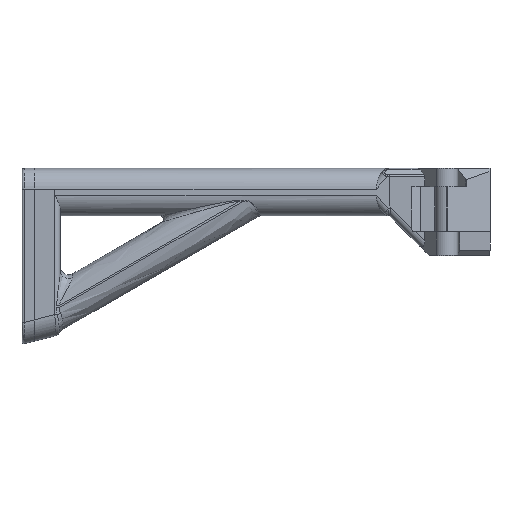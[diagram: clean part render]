
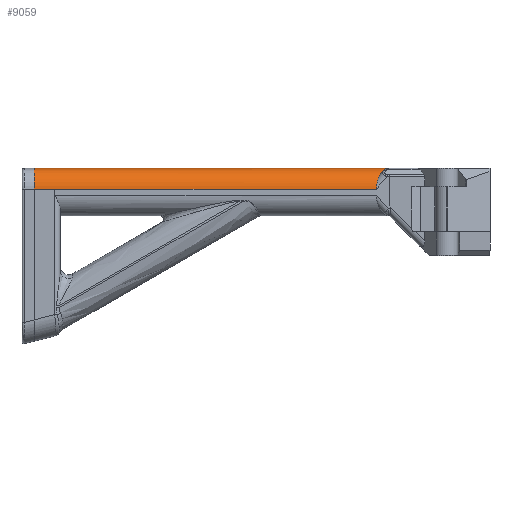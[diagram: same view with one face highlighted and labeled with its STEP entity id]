
A CAD part, top view. The second image highlights one B-rep face of the part: STEP entity #9059.
In plain terms, the highlighted cylindrical face has radius 12 mm (diameter 24 mm), a partial arc.
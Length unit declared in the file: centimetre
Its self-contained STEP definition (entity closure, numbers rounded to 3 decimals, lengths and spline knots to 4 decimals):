
#76=ELLIPSE($,#9789,1.6091,1.2);
#812=LINE($,#16482,#1668);
#829=LINE($,#16588,#1685);
#942=LINE($,#18000,#1798);
#1668=VECTOR($,#12061,18.606);
#1685=VECTOR($,#12090,20.5279);
#1798=VECTOR($,#12463,1.2);
#2109=B_SPLINE_CURVE_WITH_KNOTS($,3,(#16510,#16511,#16512,#16513,#16514,
#16515,#16516,#16517,#16518,#16519,#16520,#16521,#16522,#16523,#16524,#16525,
#16526,#16527,#16528,#16529,#16530,#16531,#16532,#16533,#16534,#16535,#16536,
#16537,#16538,#16539,#16540,#16541,#16542,#16543,#16544,#16545,#16546,#16547,
#16548,#16549,#16550,#16551,#16552,#16553,#16554,#16555,#16556,#16557),
 .UNSPECIFIED.,.F.,.F.,(4,2,2,2,2,2,2,2,2,2,2,2,2,2,2,2,2,2,2,2,2,2,2,4),
(2.2553,2.2555,2.2557,2.256,2.2565,
2.257,2.2583,2.2596,2.2621,2.2699,
2.2857,2.3174,2.3491,2.3808,2.444,
2.5071,2.5694,2.6316,2.6939,2.7562,
2.8753,2.9944,3.1135,3.2326),
 .UNSPECIFIED.);
#2110=B_SPLINE_CURVE_WITH_KNOTS($,3,(#16565,#16566,#16567,#16568,#16569,
#16570),.UNSPECIFIED.,.F.,.F.,(4,2,4),(2.7496,2.9106,
3.3544),.UNSPECIFIED.);
#2744=FACE_OUTER_BOUND($,#3293,.T.);
#3293=EDGE_LOOP($,(#8300,#8301,#8302,#8303,#8304,#8305,#8306,#8307));
#3648=CIRCLE($,#9931,1.2);
#3649=CIRCLE($,#9932,1.2);
#4307=VERTEX_POINT($,#16479);
#4308=VERTEX_POINT($,#16481);
#4315=VERTEX_POINT($,#16508);
#4316=VERTEX_POINT($,#16559);
#4317=VERTEX_POINT($,#16563);
#4325=VERTEX_POINT($,#16586);
#4456=VERTEX_POINT($,#17996);
#4458=VERTEX_POINT($,#17999);
#5508=EDGE_CURVE($,#4308,#4307,#812,.F.);
#5517=EDGE_CURVE($,#4315,#4307,#2109,.F.);
#5519=EDGE_CURVE($,#4315,#4316,#76,.F.);
#5521=EDGE_CURVE($,#4317,#4316,#2110,.F.);
#5530=EDGE_CURVE($,#4317,#4325,#829,.T.);
#5740=EDGE_CURVE($,#4458,#4456,#942,.T.);
#5757=EDGE_CURVE($,#4325,#4458,#3648,.F.);
#5758=EDGE_CURVE($,#4308,#4456,#3649,.T.);
#8300=ORIENTED_EDGE($,*,*,#5508,.T.);
#8301=ORIENTED_EDGE($,*,*,#5517,.F.);
#8302=ORIENTED_EDGE($,*,*,#5519,.T.);
#8303=ORIENTED_EDGE($,*,*,#5521,.F.);
#8304=ORIENTED_EDGE($,*,*,#5530,.T.);
#8305=ORIENTED_EDGE($,*,*,#5757,.T.);
#8306=ORIENTED_EDGE($,*,*,#5740,.T.);
#8307=ORIENTED_EDGE($,*,*,#5758,.F.);
#8557=CYLINDRICAL_SURFACE($,#9930,1.2);
#9059=ADVANCED_FACE($,(#2744),#8557,.T.);
#9789=AXIS2_PLACEMENT_3D($,#16561,#12074,#12075);
#9930=AXIS2_PLACEMENT_3D($,#18053,#12486,#12487);
#9931=AXIS2_PLACEMENT_3D($,#18054,#12488,#12489);
#9932=AXIS2_PLACEMENT_3D($,#18055,#12490,#12491);
#12061=DIRECTION($,(-1.,0.,0.));
#12074=DIRECTION('center_axis',(0.746,-0.666,0.));
#12075=DIRECTION('ref_axis',(0.666,0.746,0.));
#12090=DIRECTION($,(-1.,0.,0.));
#12463=DIRECTION($,(1.,0.,0.));
#12486=DIRECTION('center_axis',(1.,0.,0.));
#12487=DIRECTION('ref_axis',(0.,0.707,0.707));
#12488=DIRECTION('center_axis',(-1.,0.,0.));
#12489=DIRECTION('ref_axis',(0.,0.707,0.707));
#12490=DIRECTION('center_axis',(1.,0.,0.));
#12491=DIRECTION('ref_axis',(0.,0.707,0.707));
#16479=CARTESIAN_POINT('',(-26.3838,3.902,4.4797));
#16481=CARTESIAN_POINT('',(-44.9898,3.902,4.4797));
#16482=CARTESIAN_POINT($,(-46.1898,3.902,4.4797));
#16508=CARTESIAN_POINT('',(-26.1175,4.7855,4.0897));
#16510=CARTESIAN_POINT('Ctrl Pts',(-26.3838,3.902,4.4797));
#16511=CARTESIAN_POINT('Ctrl Pts',(-26.3838,3.902,4.4797));
#16512=CARTESIAN_POINT('Ctrl Pts',(-26.3839,3.902,4.4797));
#16513=CARTESIAN_POINT('Ctrl Pts',(-26.384,3.902,4.4797));
#16514=CARTESIAN_POINT('Ctrl Pts',(-26.3841,3.9021,4.4797));
#16515=CARTESIAN_POINT('Ctrl Pts',(-26.3842,3.9022,4.4797));
#16516=CARTESIAN_POINT('Ctrl Pts',(-26.3843,3.9022,4.4797));
#16517=CARTESIAN_POINT('Ctrl Pts',(-26.3844,3.9025,4.4797));
#16518=CARTESIAN_POINT('Ctrl Pts',(-26.3845,3.9027,4.4797));
#16519=CARTESIAN_POINT('Ctrl Pts',(-26.3845,3.9031,4.4797));
#16520=CARTESIAN_POINT('Ctrl Pts',(-26.3846,3.9033,4.4797));
#16521=CARTESIAN_POINT('Ctrl Pts',(-26.3846,3.9038,4.4797));
#16522=CARTESIAN_POINT('Ctrl Pts',(-26.3846,3.9043,4.4797));
#16523=CARTESIAN_POINT('Ctrl Pts',(-26.3845,3.9052,4.4797));
#16524=CARTESIAN_POINT('Ctrl Pts',(-26.3845,3.9056,4.4797));
#16525=CARTESIAN_POINT('Ctrl Pts',(-26.3844,3.907,4.4796));
#16526=CARTESIAN_POINT('Ctrl Pts',(-26.3843,3.9079,4.4796));
#16527=CARTESIAN_POINT('Ctrl Pts',(-26.3839,3.9113,4.4796));
#16528=CARTESIAN_POINT('Ctrl Pts',(-26.3835,3.9145,4.4796));
#16529=CARTESIAN_POINT('Ctrl Pts',(-26.3825,3.9223,4.4795));
#16530=CARTESIAN_POINT('Ctrl Pts',(-26.3817,3.9285,4.4793));
#16531=CARTESIAN_POINT('Ctrl Pts',(-26.3797,3.9443,4.4789));
#16532=CARTESIAN_POINT('Ctrl Pts',(-26.3781,3.9568,4.4784));
#16533=CARTESIAN_POINT('Ctrl Pts',(-26.3754,3.9777,4.4772));
#16534=CARTESIAN_POINT('Ctrl Pts',(-26.3738,3.9892,4.4764));
#16535=CARTESIAN_POINT('Ctrl Pts',(-26.3708,4.0122,4.4745));
#16536=CARTESIAN_POINT('Ctrl Pts',(-26.3692,4.0237,4.4733));
#16537=CARTESIAN_POINT('Ctrl Pts',(-26.365,4.0548,4.4698));
#16538=CARTESIAN_POINT('Ctrl Pts',(-26.3618,4.0775,4.4667));
#16539=CARTESIAN_POINT('Ctrl Pts',(-26.3552,4.1227,4.4591));
#16540=CARTESIAN_POINT('Ctrl Pts',(-26.3518,4.1451,4.4546));
#16541=CARTESIAN_POINT('Ctrl Pts',(-26.3454,4.1854,4.4454));
#16542=CARTESIAN_POINT('Ctrl Pts',(-26.3419,4.2063,4.4402));
#16543=CARTESIAN_POINT('Ctrl Pts',(-26.3345,4.2485,4.4282));
#16544=CARTESIAN_POINT('Ctrl Pts',(-26.3305,4.2699,4.4215));
#16545=CARTESIAN_POINT('Ctrl Pts',(-26.322,4.3122,4.4069));
#16546=CARTESIAN_POINT('Ctrl Pts',(-26.3175,4.3331,4.3991));
#16547=CARTESIAN_POINT('Ctrl Pts',(-26.3083,4.3734,4.3826));
#16548=CARTESIAN_POINT('Ctrl Pts',(-26.3035,4.3929,4.374));
#16549=CARTESIAN_POINT('Ctrl Pts',(-26.2896,4.4461,4.349));
#16550=CARTESIAN_POINT('Ctrl Pts',(-26.2791,4.4816,4.3302));
#16551=CARTESIAN_POINT('Ctrl Pts',(-26.255,4.5512,4.2885));
#16552=CARTESIAN_POINT('Ctrl Pts',(-26.2414,4.5853,4.2657));
#16553=CARTESIAN_POINT('Ctrl Pts',(-26.211,4.6499,4.2174));
#16554=CARTESIAN_POINT('Ctrl Pts',(-26.1941,4.6805,4.192));
#16555=CARTESIAN_POINT('Ctrl Pts',(-26.1576,4.7369,4.1407));
#16556=CARTESIAN_POINT('Ctrl Pts',(-26.138,4.7626,4.1147));
#16557=CARTESIAN_POINT('Ctrl Pts',(-26.1175,4.7855,4.0897));
#16559=CARTESIAN_POINT('',(-25.9527,4.97,3.8233));
#16561=CARTESIAN_POINT('Origin',(-26.9084,3.9002,3.2797));
#16563=CARTESIAN_POINT('',(-25.6619,5.1002,3.2797));
#16565=CARTESIAN_POINT('Ctrl Pts',(-25.9527,4.97,3.8233));
#16566=CARTESIAN_POINT('Ctrl Pts',(-25.9316,4.9936,3.7768));
#16567=CARTESIAN_POINT('Ctrl Pts',(-25.9082,5.014,3.729));
#16568=CARTESIAN_POINT('Ctrl Pts',(-25.8147,5.0785,3.5471));
#16569=CARTESIAN_POINT('Ctrl Pts',(-25.7351,5.1002,3.4082));
#16570=CARTESIAN_POINT('Ctrl Pts',(-25.6619,5.1002,3.2797));
#16586=CARTESIAN_POINT('',(-46.1898,5.1002,3.2797));
#16588=CARTESIAN_POINT($,(-46.1898,5.1002,3.2797));
#17996=CARTESIAN_POINT('',(-44.9898,3.9002,4.4797));
#17999=CARTESIAN_POINT('',(-46.1898,3.9002,4.4797));
#18000=CARTESIAN_POINT($,(-46.1898,3.9002,4.4797));
#18053=CARTESIAN_POINT('Origin',(-46.1898,3.9002,3.2797));
#18054=CARTESIAN_POINT('Origin',(-46.1898,3.9002,3.2797));
#18055=CARTESIAN_POINT('Origin',(-44.9898,3.9002,3.2797));
